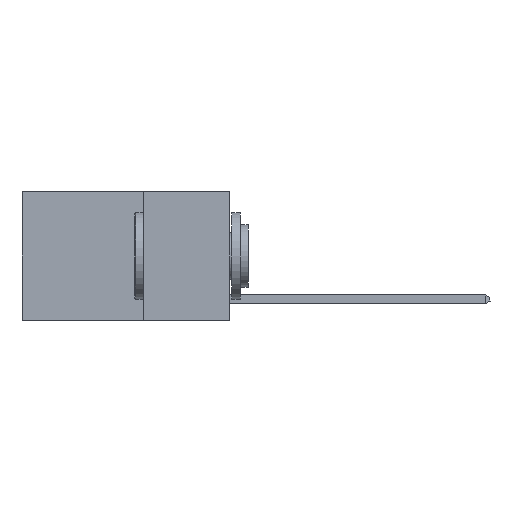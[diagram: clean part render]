
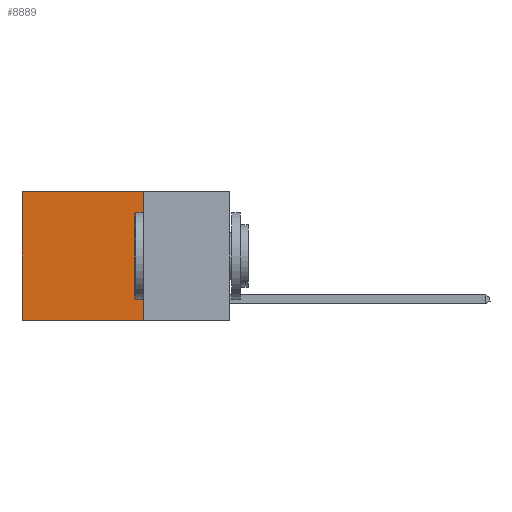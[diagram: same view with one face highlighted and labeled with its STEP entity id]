
A CAD part, left-side view. The second image highlights one B-rep face of the part: STEP entity #8889.
In plain terms, the highlighted planar face has unit normal (-1, 0, 0).
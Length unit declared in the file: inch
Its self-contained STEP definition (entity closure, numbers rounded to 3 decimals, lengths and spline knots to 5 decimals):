
#704 = LINE ( 'NONE', #12976, #16278 ) ;
#913 = ORIENTED_EDGE ( 'NONE', *, *, #1444, .F. ) ;
#1444 = EDGE_CURVE ( 'NONE', #18862, #7207, #9759, .T. ) ;
#2182 = VECTOR ( 'NONE', #7206, 39.37008 ) ;
#2348 = CARTESIAN_POINT ( 'NONE',  ( 0.2625, 0.25, 0. ) ) ;
#3187 = VERTEX_POINT ( 'NONE', #20062 ) ;
#7206 = DIRECTION ( 'NONE',  ( 0., 1., 0. ) ) ;
#7207 = VERTEX_POINT ( 'NONE', #7234 ) ;
#7234 = CARTESIAN_POINT ( 'NONE',  ( 0.2625, 0.6, -0.37 ) ) ;
#8889 = ADVANCED_FACE ( 'NONE', ( #12767 ), #11809, .F. ) ;
#8952 = LINE ( 'NONE', #20960, #13069 ) ;
#9177 = AXIS2_PLACEMENT_3D ( 'NONE', #21194, #9731, #23093 ) ;
#9731 = DIRECTION ( 'NONE',  ( 1., 0., 0. ) ) ;
#9757 = ORIENTED_EDGE ( 'NONE', *, *, #21143, .T. ) ;
#9759 = LINE ( 'NONE', #20314, #2182 ) ;
#11247 = DIRECTION ( 'NONE',  ( 0., 0., -1. ) ) ;
#11809 = PLANE ( 'NONE',  #9177 ) ;
#11854 = VERTEX_POINT ( 'NONE', #19239 ) ;
#12767 = FACE_OUTER_BOUND ( 'NONE', #14744, .T. ) ;
#12976 = CARTESIAN_POINT ( 'NONE',  ( 0.2625, 0.6, 0. ) ) ;
#13069 = VECTOR ( 'NONE', #16970, 39.37008 ) ;
#13762 = DIRECTION ( 'NONE',  ( 0., 0., -1. ) ) ;
#14744 = EDGE_LOOP ( 'NONE', ( #9757, #913, #21487, #18475 ) ) ;
#16278 = VECTOR ( 'NONE', #11247, 39.37008 ) ;
#16970 = DIRECTION ( 'NONE',  ( 0., 1., 0. ) ) ;
#17266 = VECTOR ( 'NONE', #13762, 39.37008 ) ;
#18424 = EDGE_CURVE ( 'NONE', #3187, #18862, #20477, .T. ) ;
#18475 = ORIENTED_EDGE ( 'NONE', *, *, #20156, .T. ) ;
#18862 = VERTEX_POINT ( 'NONE', #21261 ) ;
#19239 = CARTESIAN_POINT ( 'NONE',  ( 0.2625, 0.6, 0. ) ) ;
#20062 = CARTESIAN_POINT ( 'NONE',  ( 0.2625, 0.25, 0. ) ) ;
#20156 = EDGE_CURVE ( 'NONE', #3187, #11854, #8952, .T. ) ;
#20314 = CARTESIAN_POINT ( 'NONE',  ( 0.2625, 0.25, -0.37 ) ) ;
#20477 = LINE ( 'NONE', #2348, #17266 ) ;
#20960 = CARTESIAN_POINT ( 'NONE',  ( 0.2625, 0.25, 0. ) ) ;
#21143 = EDGE_CURVE ( 'NONE', #11854, #7207, #704, .T. ) ;
#21194 = CARTESIAN_POINT ( 'NONE',  ( 0.2625, 0.25, 0. ) ) ;
#21261 = CARTESIAN_POINT ( 'NONE',  ( 0.2625, 0.25, -0.37 ) ) ;
#21487 = ORIENTED_EDGE ( 'NONE', *, *, #18424, .F. ) ;
#23093 = DIRECTION ( 'NONE',  ( 0., 0., -1. ) ) ;
